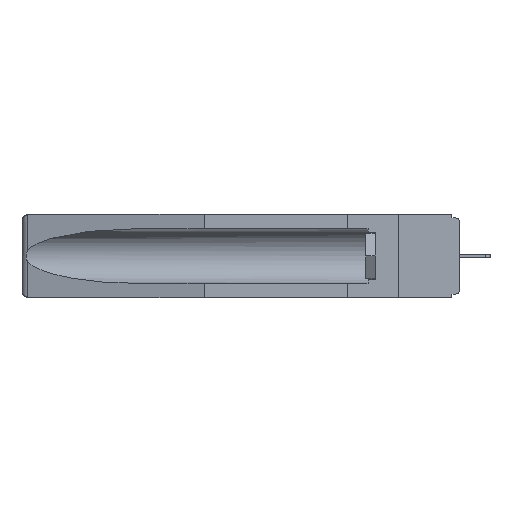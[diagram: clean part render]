
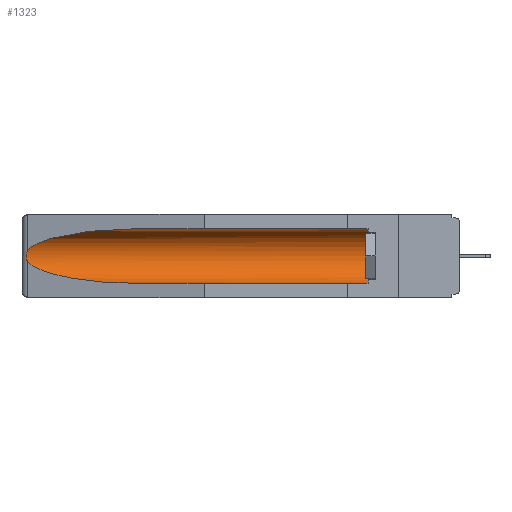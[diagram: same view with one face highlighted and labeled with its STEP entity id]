
A CAD part, left-side view. The second image highlights one B-rep face of the part: STEP entity #1323.
In plain terms, the highlighted cylindrical face has radius 2.857 mm (diameter 5.715 mm), a partial arc.
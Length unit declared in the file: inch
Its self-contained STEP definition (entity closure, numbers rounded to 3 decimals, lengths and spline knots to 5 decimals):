
#612 = VERTEX_POINT ( 'NONE', #11208 ) ;
#692 = EDGE_CURVE ( 'NONE', #612, #2253, #12018, .T. ) ;
#810 = DIRECTION ( 'NONE',  ( 0., 1., 0. ) ) ;
#1094 = CARTESIAN_POINT ( 'NONE',  ( 0.26597, 1.52961, -0.15275 ) ) ;
#1323 = ADVANCED_FACE ( 'NONE', ( #4693 ), #8540, .F. ) ;
#1681 = ORIENTED_EDGE ( 'NONE', *, *, #19457, .T. ) ;
#1751 = ORIENTED_EDGE ( 'NONE', *, *, #4406, .T. ) ;
#2253 = VERTEX_POINT ( 'NONE', #12392 ) ;
#2512 = CARTESIAN_POINT ( 'NONE',  ( 0.21114, 1.30732, -0.059 ) ) ;
#2700 = ORIENTED_EDGE ( 'NONE', *, *, #14095, .T. ) ;
#2747 = CARTESIAN_POINT ( 'NONE',  ( 0.2673, 1.5327, -0.16383 ) ) ;
#2962 = CARTESIAN_POINT ( 'NONE',  ( 0.26537, 1.52718, -0.19328 ) ) ;
#3957 = CARTESIAN_POINT ( 'NONE',  ( 0.26537, 1.52718, -0.19328 ) ) ;
#4105 = DIRECTION ( 'NONE',  ( 0., -1., 0. ) ) ;
#4376 = CARTESIAN_POINT ( 'NONE',  ( 0.2675, 1.53308, -0.17534 ) ) ;
#4406 = EDGE_CURVE ( 'NONE', #2253, #12760, #7988, .T. ) ;
#4693 = FACE_OUTER_BOUND ( 'NONE', #19469, .T. ) ;
#5999 = CARTESIAN_POINT ( 'NONE',  ( 0.26655, 1.53094, -0.18657 ) ) ;
#6702 = CARTESIAN_POINT ( 'NONE',  ( 0.155, 0.126, -0.284 ) ) ;
#6908 = VECTOR ( 'NONE', #810, 39.37008 ) ;
#7430 = CIRCLE ( 'NONE', #11117, 0.1125 ) ;
#7513 = DIRECTION ( 'NONE',  ( 0., 1., 0. ) ) ;
#7671 = CARTESIAN_POINT ( 'NONE',  ( 0.26537, 1.52718, -0.19328 ) ) ;
#7679 = EDGE_CURVE ( 'NONE', #9272, #612, #7430, .T. ) ;
#7683 = EDGE_CURVE ( 'NONE', #9272, #11813, #16909, .T. ) ;
#7988 =( BOUNDED_CURVE ( )  B_SPLINE_CURVE ( 3, ( #19303, #2512, #11541, #11947 ),
 .UNSPECIFIED., .F., .T. ) 
 B_SPLINE_CURVE_WITH_KNOTS ( ( 4, 4 ),
 ( 4.71239, 6.08839 ),
 .UNSPECIFIED. ) 
 CURVE ( )  GEOMETRIC_REPRESENTATION_ITEM ( )  RATIONAL_B_SPLINE_CURVE ( ( 1., 0.848, 0.848, 1. ) ) 
 REPRESENTATION_ITEM ( '' )  );
#8216 = CARTESIAN_POINT ( 'NONE',  ( 0.155, -0.30754, -0.1715 ) ) ;
#8540 = CYLINDRICAL_SURFACE ( 'NONE', #14520, 0.1125 ) ;
#8875 = CARTESIAN_POINT ( 'NONE',  ( 0.21114, 1.30732, -0.284 ) ) ;
#8883 = ORIENTED_EDGE ( 'NONE', *, *, #7679, .T. ) ;
#9272 = VERTEX_POINT ( 'NONE', #6702 ) ;
#10968 = ORIENTED_EDGE ( 'NONE', *, *, #692, .T. ) ;
#11117 = AXIS2_PLACEMENT_3D ( 'NONE', #13740, #4105, #15342 ) ;
#11208 = CARTESIAN_POINT ( 'NONE',  ( 0.155, 0.126, -0.059 ) ) ;
#11339 = DIRECTION ( 'NONE',  ( 0., 0., 1. ) ) ;
#11427 = DIRECTION ( 'NONE',  ( 0., 1., 0. ) ) ;
#11541 = CARTESIAN_POINT ( 'NONE',  ( 0.25451, 1.48313, -0.09465 ) ) ;
#11813 = VERTEX_POINT ( 'NONE', #18317 ) ;
#11947 = CARTESIAN_POINT ( 'NONE',  ( 0.26537, 1.52718, -0.14972 ) ) ;
#12018 = LINE ( 'NONE', #12513, #19906 ) ;
#12392 = CARTESIAN_POINT ( 'NONE',  ( 0.155, 1.07973, -0.059 ) ) ;
#12397 = CARTESIAN_POINT ( 'NONE',  ( 0.26654, 1.53092, -0.15636 ) ) ;
#12513 = CARTESIAN_POINT ( 'NONE',  ( 0.155, -0.30754, -0.059 ) ) ;
#12684 = CARTESIAN_POINT ( 'NONE',  ( 0.26537, 1.52718, -0.14972 ) ) ;
#12760 = VERTEX_POINT ( 'NONE', #12684 ) ;
#13302 = B_SPLINE_CURVE_WITH_KNOTS ( 'NONE', 3,
 ( #20230, #1094, #12397, #2747, #14014, #4376, #15604, #5999, #17203, #7671 ),
 .UNSPECIFIED., .F., .F.,
 ( 4, 2, 2, 2, 4 ),
 ( 0., 0.00029, 0.00058, 0.00087, 0.00117 ),
 .UNSPECIFIED. ) ;
#13740 = CARTESIAN_POINT ( 'NONE',  ( 0.155, 0.126, -0.1715 ) ) ;
#14014 = CARTESIAN_POINT ( 'NONE',  ( 0.2675, 1.53308, -0.16763 ) ) ;
#14095 = EDGE_CURVE ( 'NONE', #16155, #11813, #14330, .T. ) ;
#14330 =( BOUNDED_CURVE ( )  B_SPLINE_CURVE ( 3, ( #3957, #15186, #8875, #19895 ),
 .UNSPECIFIED., .F., .T. ) 
 B_SPLINE_CURVE_WITH_KNOTS ( ( 4, 4 ),
 ( 0.1948, 1.5708 ),
 .UNSPECIFIED. ) 
 CURVE ( )  GEOMETRIC_REPRESENTATION_ITEM ( )  RATIONAL_B_SPLINE_CURVE ( ( 1., 0.848, 0.848, 1. ) ) 
 REPRESENTATION_ITEM ( '' )  );
#14520 = AXIS2_PLACEMENT_3D ( 'NONE', #8216, #11427, #11339 ) ;
#15186 = CARTESIAN_POINT ( 'NONE',  ( 0.25451, 1.48313, -0.24835 ) ) ;
#15342 = DIRECTION ( 'NONE',  ( 0., 0., 1. ) ) ;
#15604 = CARTESIAN_POINT ( 'NONE',  ( 0.2673, 1.53269, -0.17917 ) ) ;
#16155 = VERTEX_POINT ( 'NONE', #2962 ) ;
#16909 = LINE ( 'NONE', #16948, #6908 ) ;
#16948 = CARTESIAN_POINT ( 'NONE',  ( 0.155, -0.30754, -0.284 ) ) ;
#17203 = CARTESIAN_POINT ( 'NONE',  ( 0.26597, 1.5296, -0.19026 ) ) ;
#18135 = ORIENTED_EDGE ( 'NONE', *, *, #7683, .F. ) ;
#18317 = CARTESIAN_POINT ( 'NONE',  ( 0.155, 1.07973, -0.284 ) ) ;
#19303 = CARTESIAN_POINT ( 'NONE',  ( 0.155, 1.07973, -0.059 ) ) ;
#19457 = EDGE_CURVE ( 'NONE', #12760, #16155, #13302, .T. ) ;
#19469 = EDGE_LOOP ( 'NONE', ( #1751, #1681, #2700, #18135, #8883, #10968 ) ) ;
#19895 = CARTESIAN_POINT ( 'NONE',  ( 0.155, 1.07973, -0.284 ) ) ;
#19906 = VECTOR ( 'NONE', #7513, 39.37008 ) ;
#20230 = CARTESIAN_POINT ( 'NONE',  ( 0.26537, 1.52718, -0.14972 ) ) ;
